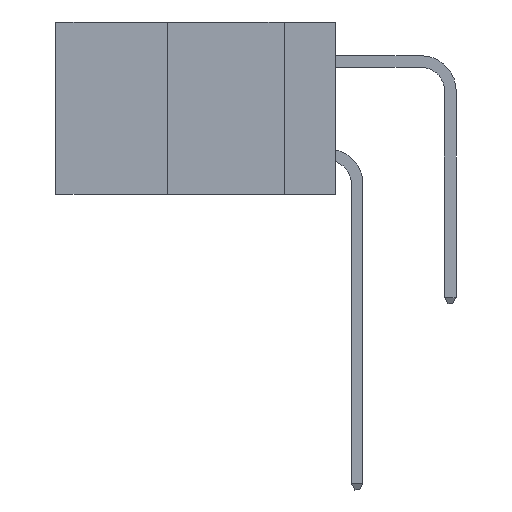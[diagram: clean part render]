
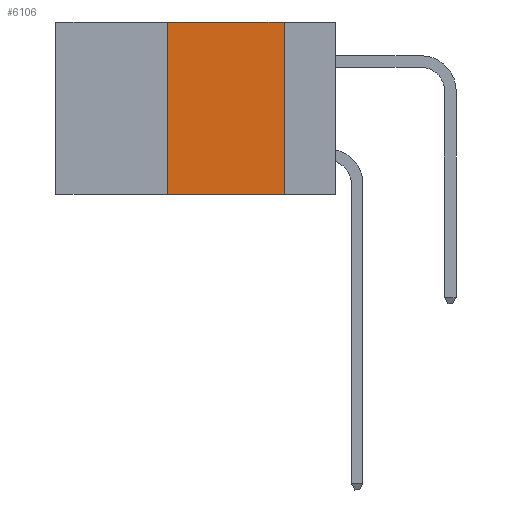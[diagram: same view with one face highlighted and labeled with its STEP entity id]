
A CAD part, left-side view. The second image highlights one B-rep face of the part: STEP entity #6106.
In plain terms, the highlighted planar face has unit normal (-1, 0, 0).
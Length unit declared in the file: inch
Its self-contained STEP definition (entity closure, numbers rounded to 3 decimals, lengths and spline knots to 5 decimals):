
#290 = EDGE_CURVE ( 'NONE', #18543, #6486, #22693, .T. ) ;
#4921 = VECTOR ( 'NONE', #8792, 39.37008 ) ;
#5218 = CARTESIAN_POINT ( 'NONE',  ( 0., 0.6, 0. ) ) ;
#5942 = EDGE_LOOP ( 'NONE', ( #27834, #26411, #26197, #27539 ) ) ;
#6106 = ADVANCED_FACE ( 'NONE', ( #22870 ), #18792, .F. ) ;
#6486 = VERTEX_POINT ( 'NONE', #21575 ) ;
#7234 = DIRECTION ( 'NONE',  ( 0., 0., 1. ) ) ;
#8327 = AXIS2_PLACEMENT_3D ( 'NONE', #21508, #19214, #16723 ) ;
#8792 = DIRECTION ( 'NONE',  ( 0., 0., -1. ) ) ;
#8799 = LINE ( 'NONE', #27064, #26996 ) ;
#9500 = CARTESIAN_POINT ( 'NONE',  ( 0., 0.36, -0.37 ) ) ;
#11247 = CARTESIAN_POINT ( 'NONE',  ( 0., 0.11, 0. ) ) ;
#12321 = LINE ( 'NONE', #26314, #4921 ) ;
#15134 = DIRECTION ( 'NONE',  ( 0., -1., 0. ) ) ;
#16360 = EDGE_CURVE ( 'NONE', #18735, #27671, #20870, .T. ) ;
#16723 = DIRECTION ( 'NONE',  ( 0., 0., -1. ) ) ;
#17081 = EDGE_CURVE ( 'NONE', #27671, #6486, #12321, .T. ) ;
#18543 = VERTEX_POINT ( 'NONE', #9500 ) ;
#18735 = VERTEX_POINT ( 'NONE', #20891 ) ;
#18792 = PLANE ( 'NONE',  #8327 ) ;
#19214 = DIRECTION ( 'NONE',  ( 1., 0., 0. ) ) ;
#19530 = DIRECTION ( 'NONE',  ( 0., -1., 0. ) ) ;
#20870 = LINE ( 'NONE', #5218, #22028 ) ;
#20891 = CARTESIAN_POINT ( 'NONE',  ( 0., 0.36, 0. ) ) ;
#21508 = CARTESIAN_POINT ( 'NONE',  ( 0., 0.6, 0. ) ) ;
#21575 = CARTESIAN_POINT ( 'NONE',  ( 0., 0.11, -0.37 ) ) ;
#22028 = VECTOR ( 'NONE', #19530, 39.37008 ) ;
#22693 = LINE ( 'NONE', #25071, #24253 ) ;
#22870 = FACE_OUTER_BOUND ( 'NONE', #5942, .T. ) ;
#24253 = VECTOR ( 'NONE', #15134, 39.37008 ) ;
#25071 = CARTESIAN_POINT ( 'NONE',  ( 0., 0.6, -0.37 ) ) ;
#26197 = ORIENTED_EDGE ( 'NONE', *, *, #31242, .F. ) ;
#26314 = CARTESIAN_POINT ( 'NONE',  ( 0., 0.11, 0. ) ) ;
#26411 = ORIENTED_EDGE ( 'NONE', *, *, #16360, .F. ) ;
#26996 = VECTOR ( 'NONE', #7234, 39.37008 ) ;
#27064 = CARTESIAN_POINT ( 'NONE',  ( 0., 0.36, 0. ) ) ;
#27539 = ORIENTED_EDGE ( 'NONE', *, *, #290, .T. ) ;
#27671 = VERTEX_POINT ( 'NONE', #11247 ) ;
#27834 = ORIENTED_EDGE ( 'NONE', *, *, #17081, .F. ) ;
#31242 = EDGE_CURVE ( 'NONE', #18543, #18735, #8799, .T. ) ;
